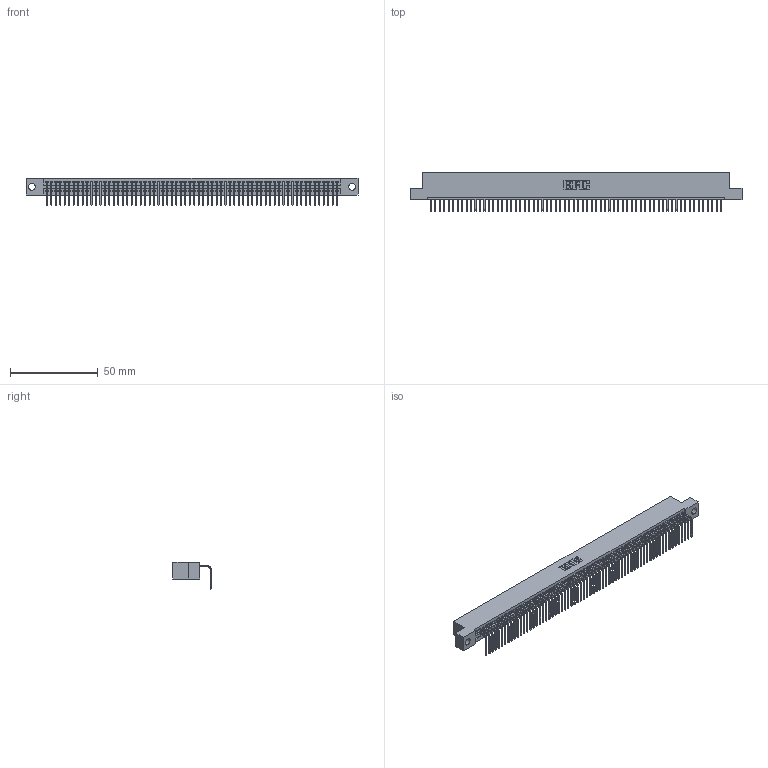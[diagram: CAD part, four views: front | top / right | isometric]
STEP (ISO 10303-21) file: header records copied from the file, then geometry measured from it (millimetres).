
FILE_DESCRIPTION (( 'STEP AP203' ), '1' );
FILE_NAME ('345-066-558-104.STEP', '2021-06-10T15:13:02', ( '' ), ( '' ), 'SwSTEP 2.0', 'SolidWorks 2020', '' );
FILE_SCHEMA (( 'CONFIG_CONTROL_DESIGN' ));
Length unit declared in the file: inch
Products named in the file (3): 345-066-558-104; 345-292-001_558 Tail - 2; 345 Part_Flush Mounting Lugs - 0.156 Dia-TI
Assembly tree (67 placements, depth 2):
  345-066-558-104
    345 Part_Flush Mounting Lugs - 0.156 Dia-TI
    345-292-001_558 Tail - 2  x66
Bounding box: 188.85 x 21.83 x 15.37 mm (x, y, z)
Volume: 18247.6 mm3; surface area: 25710.2 mm2
Topology: 67 solids, 67 shells, 4100 faces, 12389 edges, 8170 vertices
Faces by surface type: plane 2866, cylinder 1234
Entity records: 46945 total; most frequent: CARTESIAN_POINT 8140, ORIENTED_EDGE 8138, DIRECTION 7073, EDGE_CURVE 4069, VECTOR 3673, LINE 3673, VERTEX_POINT 2710, AXIS2_PLACEMENT_3D 1700
